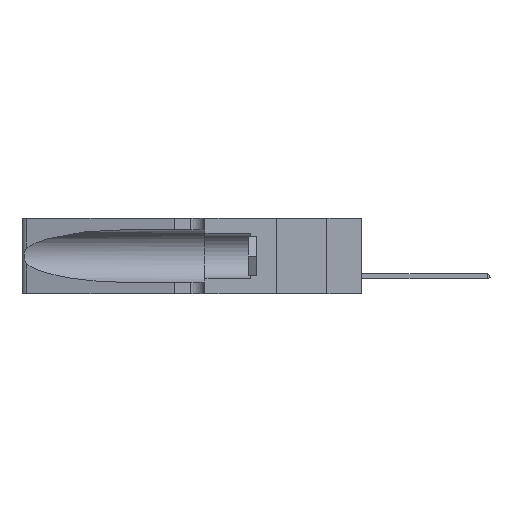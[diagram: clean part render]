
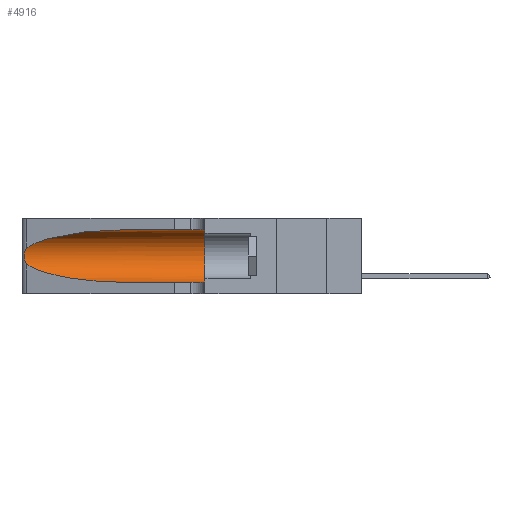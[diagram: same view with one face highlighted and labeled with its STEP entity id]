
A CAD part, left-side view. The second image highlights one B-rep face of the part: STEP entity #4916.
In plain terms, the highlighted cylindrical face has radius 3.308 mm (diameter 6.617 mm), a partial arc.
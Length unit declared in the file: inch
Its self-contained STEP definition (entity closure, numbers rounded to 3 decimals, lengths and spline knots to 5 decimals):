
#474 =( BOUNDED_CURVE ( )  B_SPLINE_CURVE ( 3, ( #23885, #6737, #1134, #2869 ),
 .UNSPECIFIED., .F., .T. ) 
 B_SPLINE_CURVE_WITH_KNOTS ( ( 4, 4 ),
 ( 1.5708, 2.84003 ),
 .UNSPECIFIED. ) 
 CURVE ( )  GEOMETRIC_REPRESENTATION_ITEM ( )  RATIONAL_B_SPLINE_CURVE ( ( 1., 0.87, 0.87, 1. ) ) 
 REPRESENTATION_ITEM ( '' )  );
#488 = AXIS2_PLACEMENT_3D ( 'NONE', #21002, #17240, #21086 ) ;
#805 = CARTESIAN_POINT ( 'NONE',  ( 0.1305, 0.35, 0.31525 ) ) ;
#1134 = CARTESIAN_POINT ( 'NONE',  ( 0.2373, 1.15595, 0.28018 ) ) ;
#2048 = EDGE_LOOP ( 'NONE', ( #8592, #11899, #5703, #14974, #4536, #23486 ) ) ;
#2059 = CARTESIAN_POINT ( 'NONE',  ( 0.25487, 1.22718, 0.22369 ) ) ;
#2279 = CARTESIAN_POINT ( 'NONE',  ( 0.25856, 1.23593, 0.16098 ) ) ;
#2869 = CARTESIAN_POINT ( 'NONE',  ( 0.25487, 1.22718, 0.22369 ) ) ;
#3890 = CARTESIAN_POINT ( 'NONE',  ( 0.1305, 0.72297, 0.05475 ) ) ;
#4536 = ORIENTED_EDGE ( 'NONE', *, *, #12621, .F. ) ;
#4727 = VERTEX_POINT ( 'NONE', #5265 ) ;
#4916 = ADVANCED_FACE ( 'NONE', ( #8453 ), #12055, .F. ) ;
#5265 = CARTESIAN_POINT ( 'NONE',  ( 0.1305, 0.72297, 0.05475 ) ) ;
#5658 = CARTESIAN_POINT ( 'NONE',  ( 0.26075, 1.23896, 0.19203 ) ) ;
#5703 = ORIENTED_EDGE ( 'NONE', *, *, #9276, .T. ) ;
#5758 = EDGE_CURVE ( 'NONE', #23082, #13189, #9637, .T. ) ;
#6737 = CARTESIAN_POINT ( 'NONE',  ( 0.18966, 0.96281, 0.31525 ) ) ;
#6787 = AXIS2_PLACEMENT_3D ( 'NONE', #15261, #7798, #7879 ) ;
#7798 = DIRECTION ( 'NONE',  ( 0., -1., 0. ) ) ;
#7879 = DIRECTION ( 'NONE',  ( 0., 0., -1. ) ) ;
#7940 = CARTESIAN_POINT ( 'NONE',  ( 0.25555, 1.22993, 0.14849 ) ) ;
#8287 = CARTESIAN_POINT ( 'NONE',  ( 0.1305, 0.72297, 0.31525 ) ) ;
#8453 = FACE_OUTER_BOUND ( 'NONE', #2048, .T. ) ;
#8491 = CARTESIAN_POINT ( 'NONE',  ( 0.25487, 1.22718, 0.14631 ) ) ;
#8592 = ORIENTED_EDGE ( 'NONE', *, *, #19122, .T. ) ;
#8604 =( BOUNDED_CURVE ( )  B_SPLINE_CURVE ( 3, ( #20507, #12784, #11187, #3890 ),
 .UNSPECIFIED., .F., .F. ) 
 B_SPLINE_CURVE_WITH_KNOTS ( ( 4, 4 ),
 ( 3.44316, 4.71239 ),
 .UNSPECIFIED. ) 
 CURVE ( )  GEOMETRIC_REPRESENTATION_ITEM ( )  RATIONAL_B_SPLINE_CURVE ( ( 1., 0.87, 0.87, 1. ) ) 
 REPRESENTATION_ITEM ( '' )  );
#8840 = VERTEX_POINT ( 'NONE', #8491 ) ;
#9276 = EDGE_CURVE ( 'NONE', #8840, #4727, #8604, .T. ) ;
#9637 = LINE ( 'NONE', #10820, #23013 ) ;
#9684 = VERTEX_POINT ( 'NONE', #21752 ) ;
#9857 = CARTESIAN_POINT ( 'NONE',  ( 0.26017, 1.23833, 0.17102 ) ) ;
#10820 = CARTESIAN_POINT ( 'NONE',  ( 0.1305, 1.61858, 0.31525 ) ) ;
#11187 = CARTESIAN_POINT ( 'NONE',  ( 0.18966, 0.96281, 0.05475 ) ) ;
#11641 = VERTEX_POINT ( 'NONE', #17559 ) ;
#11659 = B_SPLINE_CURVE_WITH_KNOTS ( 'NONE', 3,
 ( #2059, #17065, #15082, #16980, #15393, #18905, #5658, #13662, #9857, #2279, #19551, #15635, #7940, #23390 ),
 .UNSPECIFIED., .F., .F.,
 ( 4, 2, 2, 2, 2, 2, 4 ),
 ( 0., 0.00027, 0.00053, 0.00107, 0.0016, 0.00187, 0.00214 ),
 .UNSPECIFIED. ) ;
#11899 = ORIENTED_EDGE ( 'NONE', *, *, #21001, .T. ) ;
#12055 = CYLINDRICAL_SURFACE ( 'NONE', #6787, 0.13025 ) ;
#12621 = EDGE_CURVE ( 'NONE', #13189, #9684, #14027, .T. ) ;
#12784 = CARTESIAN_POINT ( 'NONE',  ( 0.2373, 1.15595, 0.08982 ) ) ;
#13189 = VERTEX_POINT ( 'NONE', #805 ) ;
#13662 = CARTESIAN_POINT ( 'NONE',  ( 0.26075, 1.23896, 0.178 ) ) ;
#14027 = CIRCLE ( 'NONE', #488, 0.13025 ) ;
#14974 = ORIENTED_EDGE ( 'NONE', *, *, #16403, .T. ) ;
#15082 = CARTESIAN_POINT ( 'NONE',  ( 0.25639, 1.23184, 0.21858 ) ) ;
#15261 = CARTESIAN_POINT ( 'NONE',  ( 0.1305, 1.61858, 0.185 ) ) ;
#15393 = CARTESIAN_POINT ( 'NONE',  ( 0.25854, 1.2359, 0.20912 ) ) ;
#15635 = CARTESIAN_POINT ( 'NONE',  ( 0.25639, 1.23186, 0.15144 ) ) ;
#16403 = EDGE_CURVE ( 'NONE', #4727, #9684, #23280, .T. ) ;
#16980 = CARTESIAN_POINT ( 'NONE',  ( 0.25787, 1.23484, 0.2124 ) ) ;
#17065 = CARTESIAN_POINT ( 'NONE',  ( 0.25555, 1.22994, 0.2215 ) ) ;
#17240 = DIRECTION ( 'NONE',  ( 0., 1., 0. ) ) ;
#17559 = CARTESIAN_POINT ( 'NONE',  ( 0.25487, 1.22718, 0.22369 ) ) ;
#18905 = CARTESIAN_POINT ( 'NONE',  ( 0.26018, 1.23835, 0.19895 ) ) ;
#19122 = EDGE_CURVE ( 'NONE', #23082, #11641, #474, .T. ) ;
#19551 = CARTESIAN_POINT ( 'NONE',  ( 0.25789, 1.23486, 0.15765 ) ) ;
#20425 = DIRECTION ( 'NONE',  ( 0., -1., 0. ) ) ;
#20507 = CARTESIAN_POINT ( 'NONE',  ( 0.25487, 1.22718, 0.14631 ) ) ;
#21001 = EDGE_CURVE ( 'NONE', #11641, #8840, #11659, .T. ) ;
#21002 = CARTESIAN_POINT ( 'NONE',  ( 0.1305, 0.35, 0.185 ) ) ;
#21086 = DIRECTION ( 'NONE',  ( 0., 0., 1. ) ) ;
#21752 = CARTESIAN_POINT ( 'NONE',  ( 0.1305, 0.35, 0.05475 ) ) ;
#21801 = VECTOR ( 'NONE', #20425, 39.37008 ) ;
#22047 = DIRECTION ( 'NONE',  ( 0., -1., 0. ) ) ;
#23013 = VECTOR ( 'NONE', #22047, 39.37008 ) ;
#23082 = VERTEX_POINT ( 'NONE', #8287 ) ;
#23280 = LINE ( 'NONE', #24347, #21801 ) ;
#23390 = CARTESIAN_POINT ( 'NONE',  ( 0.25487, 1.22718, 0.14631 ) ) ;
#23486 = ORIENTED_EDGE ( 'NONE', *, *, #5758, .F. ) ;
#23885 = CARTESIAN_POINT ( 'NONE',  ( 0.1305, 0.72297, 0.31525 ) ) ;
#24347 = CARTESIAN_POINT ( 'NONE',  ( 0.1305, 1.61858, 0.05475 ) ) ;
